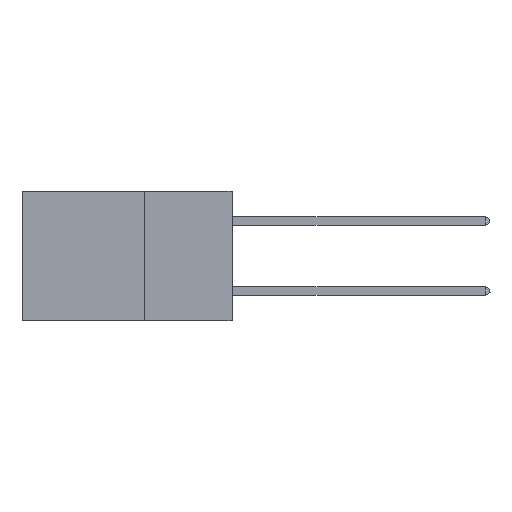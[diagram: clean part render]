
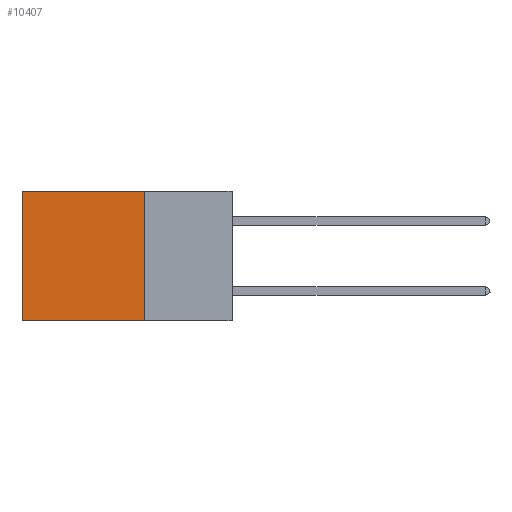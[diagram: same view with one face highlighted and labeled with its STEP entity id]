
A CAD part, left-side view. The second image highlights one B-rep face of the part: STEP entity #10407.
In plain terms, the highlighted planar face has unit normal (-1, 0, 0).
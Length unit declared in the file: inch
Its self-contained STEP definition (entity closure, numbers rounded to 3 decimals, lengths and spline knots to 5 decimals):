
#421 = PLANE ( 'NONE',  #15108 ) ;
#917 = VERTEX_POINT ( 'NONE', #9377 ) ;
#1388 = FACE_OUTER_BOUND ( 'NONE', #11340, .T. ) ;
#1763 = VERTEX_POINT ( 'NONE', #8601 ) ;
#2116 = DIRECTION ( 'NONE',  ( 1., 0., 0. ) ) ;
#2391 = VECTOR ( 'NONE', #21750, 39.37008 ) ;
#3617 = ORIENTED_EDGE ( 'NONE', *, *, #13973, .T. ) ;
#3889 = DIRECTION ( 'NONE',  ( 0., 1., 0. ) ) ;
#4872 = VERTEX_POINT ( 'NONE', #8387 ) ;
#5082 = DIRECTION ( 'NONE',  ( 0., 1., 0. ) ) ;
#5222 = VECTOR ( 'NONE', #19622, 39.37008 ) ;
#5911 = EDGE_CURVE ( 'NONE', #4872, #1763, #21670, .T. ) ;
#6985 = VERTEX_POINT ( 'NONE', #17943 ) ;
#7534 = EDGE_CURVE ( 'NONE', #4872, #6985, #14124, .T. ) ;
#8387 = CARTESIAN_POINT ( 'NONE',  ( 0.2875, 0.25, 0. ) ) ;
#8601 = CARTESIAN_POINT ( 'NONE',  ( 0.2875, 0.6, 0. ) ) ;
#9089 = CARTESIAN_POINT ( 'NONE',  ( 0.2875, 0.25, 0. ) ) ;
#9139 = ORIENTED_EDGE ( 'NONE', *, *, #7534, .F. ) ;
#9377 = CARTESIAN_POINT ( 'NONE',  ( 0.2875, 0.6, -0.37 ) ) ;
#10407 = ADVANCED_FACE ( 'NONE', ( #1388 ), #421, .F. ) ;
#10757 = LINE ( 'NONE', #16658, #16311 ) ;
#10810 = VECTOR ( 'NONE', #3889, 39.37008 ) ;
#10978 = ORIENTED_EDGE ( 'NONE', *, *, #11532, .F. ) ;
#11340 = EDGE_LOOP ( 'NONE', ( #3617, #10978, #9139, #14238 ) ) ;
#11532 = EDGE_CURVE ( 'NONE', #6985, #917, #10757, .T. ) ;
#11546 = LINE ( 'NONE', #14140, #2391 ) ;
#12153 = CARTESIAN_POINT ( 'NONE',  ( 0.2875, 0.25, 0. ) ) ;
#13973 = EDGE_CURVE ( 'NONE', #1763, #917, #11546, .T. ) ;
#14124 = LINE ( 'NONE', #20317, #5222 ) ;
#14140 = CARTESIAN_POINT ( 'NONE',  ( 0.2875, 0.6, 0. ) ) ;
#14238 = ORIENTED_EDGE ( 'NONE', *, *, #5911, .T. ) ;
#15108 = AXIS2_PLACEMENT_3D ( 'NONE', #12153, #2116, #15495 ) ;
#15495 = DIRECTION ( 'NONE',  ( 0., 0., -1. ) ) ;
#16311 = VECTOR ( 'NONE', #5082, 39.37008 ) ;
#16658 = CARTESIAN_POINT ( 'NONE',  ( 0.2875, 0.25, -0.37 ) ) ;
#17943 = CARTESIAN_POINT ( 'NONE',  ( 0.2875, 0.25, -0.37 ) ) ;
#19622 = DIRECTION ( 'NONE',  ( 0., 0., -1. ) ) ;
#20317 = CARTESIAN_POINT ( 'NONE',  ( 0.2875, 0.25, 0. ) ) ;
#21670 = LINE ( 'NONE', #9089, #10810 ) ;
#21750 = DIRECTION ( 'NONE',  ( 0., 0., -1. ) ) ;
